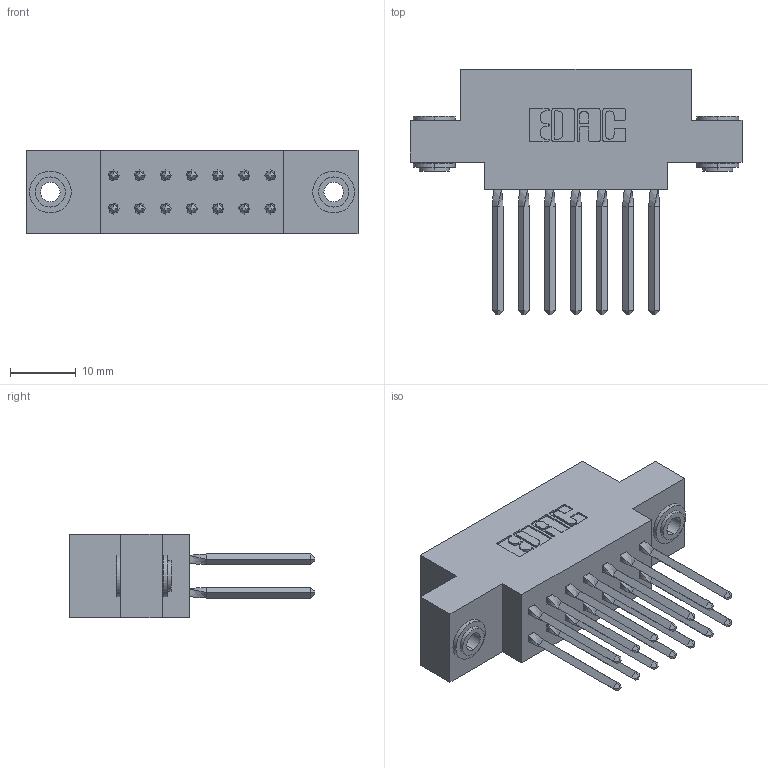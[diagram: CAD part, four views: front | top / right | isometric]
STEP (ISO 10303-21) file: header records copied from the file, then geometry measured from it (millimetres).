
FILE_DESCRIPTION (( 'STEP AP203' ), '1' );
FILE_NAME ('317-014-540-803.STEP', '2020-02-27T14:42:01', ( '' ), ( '' ), 'SwSTEP 2.0', 'SolidWorks 2016', '' );
FILE_SCHEMA (( 'CONFIG_CONTROL_DESIGN' ));
Length unit declared in the file: inch
Products named in the file (4): 345-250-002_345-250-002-102; 317-014-540-803; 317-290-001_540; 317 Part_.156 Dia - TH
Assembly tree (17 placements, depth 2):
  317-014-540-803
    317 Part_.156 Dia - TH
    317-290-001_540  x14
    345-250-002_345-250-002-102  x2
Bounding box: 50.44 x 37.34 x 12.7 mm (x, y, z)
Volume: 7302.1 mm3; surface area: 9778.1 mm2
Topology: 17 solids, 17 shells, 1386 faces, 3809 edges, 2456 vertices
Faces by surface type: plane 1090, cylinder 232, bspline 56, cone 8
Entity records: 15651 total; most frequent: CARTESIAN_POINT 3110, ORIENTED_EDGE 2602, DIRECTION 2217, EDGE_CURVE 1301, LINE 1021, VECTOR 1021, VERTEX_POINT 859, AXIS2_PLACEMENT_3D 598
